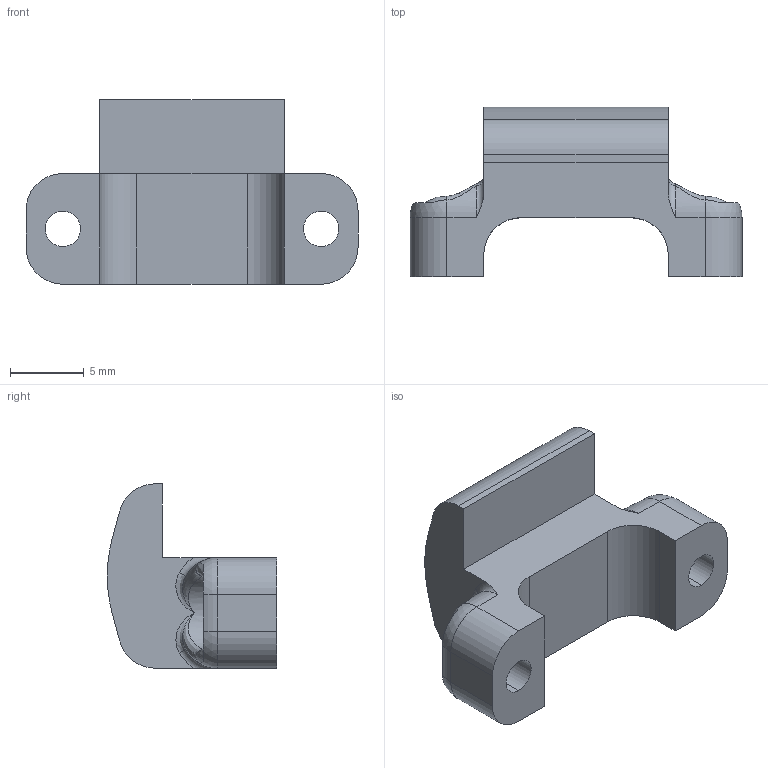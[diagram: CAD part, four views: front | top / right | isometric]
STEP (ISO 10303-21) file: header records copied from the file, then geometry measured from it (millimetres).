
FILE_DESCRIPTION (( 'STEP AP203' ), '1' );
FILE_NAME ('Trigger_Guide.STEP', '2013-11-10T07:43:56', ( '' ), ( '' ), 'SwSTEP 2.0', 'SolidWorks 2013', '' );
FILE_SCHEMA (( 'CONFIG_CONTROL_DESIGN' ));
Length unit declared in the file: millimetre
Products named in the file (1): Trigger_Guide
Bounding box: 22.5 x 11.5 x 12.5 mm (x, y, z)
Volume: 1169.5 mm3; surface area: 971.5 mm2
Topology: 1 solids, 1 shells, 60 faces, 155 edges, 93 vertices
Faces by surface type: cylinder 23, plane 17, bspline 12, sphere 4, torus 4
Entity records: 2643 total; most frequent: CARTESIAN_POINT 1185, ORIENTED_EDGE 302, DIRECTION 276, EDGE_CURVE 151, AXIS2_PLACEMENT_3D 108, VERTEX_POINT 93, EDGE_LOOP 64, FACE_OUTER_BOUND 60
